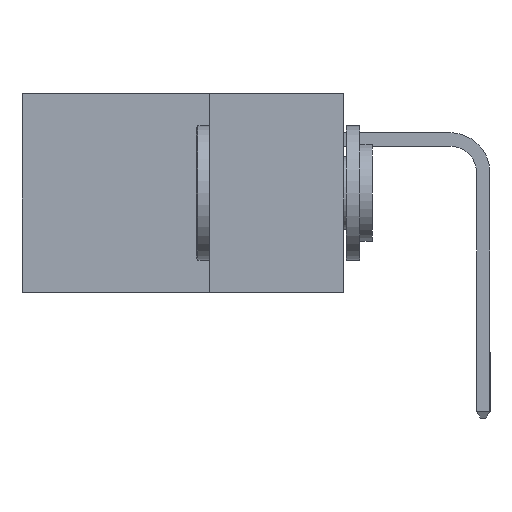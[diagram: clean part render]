
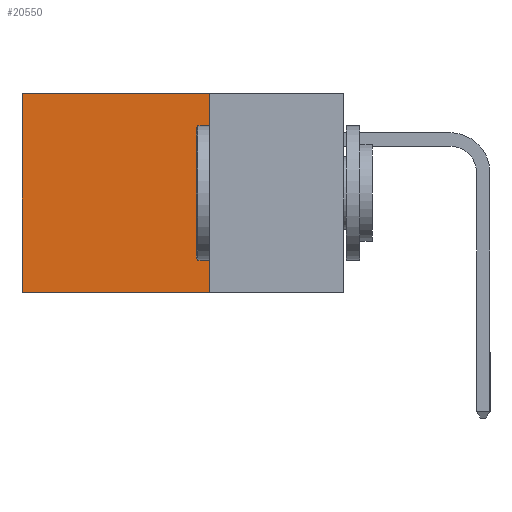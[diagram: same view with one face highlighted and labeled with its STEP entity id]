
A CAD part, left-side view. The second image highlights one B-rep face of the part: STEP entity #20550.
In plain terms, the highlighted planar face has unit normal (-1, 0, 0).
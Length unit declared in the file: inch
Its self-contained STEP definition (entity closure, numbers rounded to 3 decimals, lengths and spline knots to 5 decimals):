
#223 = VECTOR ( 'NONE', #3085, 39.37008 ) ;
#323 = VERTEX_POINT ( 'NONE', #18436 ) ;
#680 = CARTESIAN_POINT ( 'NONE',  ( 0.298, 0.25, -0.37 ) ) ;
#2411 = DIRECTION ( 'NONE',  ( 0., 0., -1. ) ) ;
#2775 = VECTOR ( 'NONE', #4411, 39.37008 ) ;
#3085 = DIRECTION ( 'NONE',  ( 0., 0., -1. ) ) ;
#3159 = VECTOR ( 'NONE', #15632, 39.37008 ) ;
#3401 = ORIENTED_EDGE ( 'NONE', *, *, #17265, .F. ) ;
#3523 = VERTEX_POINT ( 'NONE', #6629 ) ;
#4062 = CARTESIAN_POINT ( 'NONE',  ( 0.298, 0.25, 0. ) ) ;
#4411 = DIRECTION ( 'NONE',  ( 0., 0., -1. ) ) ;
#6108 = CARTESIAN_POINT ( 'NONE',  ( 0.298, 0.6, 0. ) ) ;
#6629 = CARTESIAN_POINT ( 'NONE',  ( 0.298, 0.6, 0. ) ) ;
#7894 = VECTOR ( 'NONE', #13039, 39.37008 ) ;
#8303 = LINE ( 'NONE', #6108, #2775 ) ;
#8902 = EDGE_LOOP ( 'NONE', ( #13311, #3401, #20301, #14200 ) ) ;
#10067 = FACE_OUTER_BOUND ( 'NONE', #8902, .T. ) ;
#10880 = EDGE_CURVE ( 'NONE', #22599, #3523, #18835, .T. ) ;
#11276 = PLANE ( 'NONE',  #18241 ) ;
#12036 = LINE ( 'NONE', #13579, #223 ) ;
#12923 = DIRECTION ( 'NONE',  ( 1., 0., 0. ) ) ;
#13039 = DIRECTION ( 'NONE',  ( 0., 1., 0. ) ) ;
#13311 = ORIENTED_EDGE ( 'NONE', *, *, #14295, .T. ) ;
#13318 = LINE ( 'NONE', #680, #7894 ) ;
#13579 = CARTESIAN_POINT ( 'NONE',  ( 0.298, 0.25, 0. ) ) ;
#13918 = VERTEX_POINT ( 'NONE', #22309 ) ;
#14200 = ORIENTED_EDGE ( 'NONE', *, *, #10880, .T. ) ;
#14295 = EDGE_CURVE ( 'NONE', #3523, #13918, #8303, .T. ) ;
#15632 = DIRECTION ( 'NONE',  ( 0., 1., 0. ) ) ;
#15864 = EDGE_CURVE ( 'NONE', #22599, #323, #12036, .T. ) ;
#17265 = EDGE_CURVE ( 'NONE', #323, #13918, #13318, .T. ) ;
#18241 = AXIS2_PLACEMENT_3D ( 'NONE', #4062, #12923, #2411 ) ;
#18436 = CARTESIAN_POINT ( 'NONE',  ( 0.298, 0.25, -0.37 ) ) ;
#18835 = LINE ( 'NONE', #22639, #3159 ) ;
#20301 = ORIENTED_EDGE ( 'NONE', *, *, #15864, .F. ) ;
#20550 = ADVANCED_FACE ( 'NONE', ( #10067 ), #11276, .F. ) ;
#20721 = CARTESIAN_POINT ( 'NONE',  ( 0.298, 0.25, 0. ) ) ;
#22309 = CARTESIAN_POINT ( 'NONE',  ( 0.298, 0.6, -0.37 ) ) ;
#22599 = VERTEX_POINT ( 'NONE', #20721 ) ;
#22639 = CARTESIAN_POINT ( 'NONE',  ( 0.298, 0.25, 0. ) ) ;
